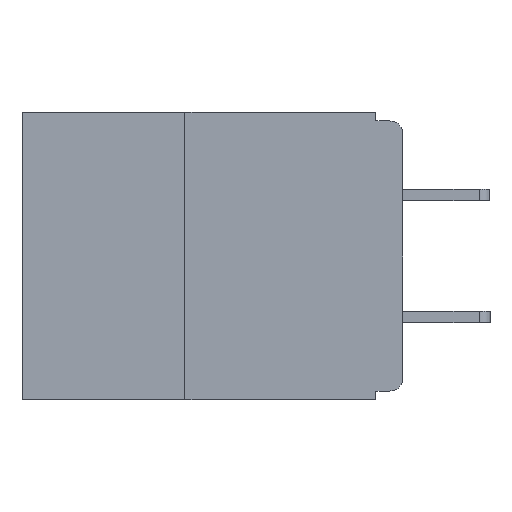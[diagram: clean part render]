
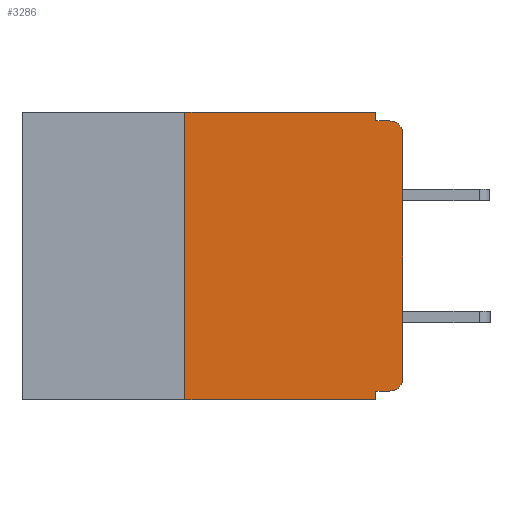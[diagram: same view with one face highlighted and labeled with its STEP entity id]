
A CAD part, left-side view. The second image highlights one B-rep face of the part: STEP entity #3286.
In plain terms, the highlighted planar face has unit normal (-1, 0, 0).
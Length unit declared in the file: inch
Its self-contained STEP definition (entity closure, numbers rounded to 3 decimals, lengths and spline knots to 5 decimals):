
#196 = CARTESIAN_POINT ( 'NONE',  ( 0., 0.031, 0. ) ) ;
#295 = EDGE_CURVE ( 'NONE', #16377, #27102, #6741, .T. ) ;
#444 = EDGE_CURVE ( 'NONE', #8592, #17327, #26393, .T. ) ;
#809 = DIRECTION ( 'NONE',  ( -1., 0., 0. ) ) ;
#1293 = VERTEX_POINT ( 'NONE', #15993 ) ;
#1761 = EDGE_CURVE ( 'NONE', #8592, #17050, #13873, .T. ) ;
#3118 = ORIENTED_EDGE ( 'NONE', *, *, #4079, .T. ) ;
#3286 = ADVANCED_FACE ( 'NONE', ( #9247 ), #17179, .F. ) ;
#4079 = EDGE_CURVE ( 'NONE', #17050, #16705, #19885, .T. ) ;
#4694 = ORIENTED_EDGE ( 'NONE', *, *, #1761, .T. ) ;
#5851 = CARTESIAN_POINT ( 'NONE',  ( 0., 0., 0. ) ) ;
#6332 = CARTESIAN_POINT ( 'NONE',  ( 0., 0., -0.025 ) ) ;
#6379 = CARTESIAN_POINT ( 'NONE',  ( 0., 0., -0.01 ) ) ;
#6396 = DIRECTION ( 'NONE',  ( 0., 0., -1. ) ) ;
#6573 = DIRECTION ( 'NONE',  ( 1., 0., 0. ) ) ;
#6720 = EDGE_LOOP ( 'NONE', ( #3118, #16031, #24712, #26273, #27797, #9269, #13804, #28202, #9662, #4694 ) ) ;
#6741 = LINE ( 'NONE', #27504, #24470 ) ;
#7081 = EDGE_CURVE ( 'NONE', #17327, #18658, #19704, .T. ) ;
#7130 = VERTEX_POINT ( 'NONE', #9991 ) ;
#7249 = VECTOR ( 'NONE', #15002, 39.37008 ) ;
#8592 = VERTEX_POINT ( 'NONE', #11400 ) ;
#9129 = CARTESIAN_POINT ( 'NONE',  ( 0., 0.031, -0.33 ) ) ;
#9247 = FACE_OUTER_BOUND ( 'NONE', #6720, .T. ) ;
#9269 = ORIENTED_EDGE ( 'NONE', *, *, #17254, .F. ) ;
#9607 = DIRECTION ( 'NONE',  ( 0., 0., -1. ) ) ;
#9662 = ORIENTED_EDGE ( 'NONE', *, *, #444, .F. ) ;
#9991 = CARTESIAN_POINT ( 'NONE',  ( 0., 0.015, -0.01 ) ) ;
#11129 = EDGE_CURVE ( 'NONE', #27102, #7130, #21011, .T. ) ;
#11400 = CARTESIAN_POINT ( 'NONE',  ( 0., 0.015, -0.32 ) ) ;
#11452 = VECTOR ( 'NONE', #14889, 39.37008 ) ;
#12587 = CARTESIAN_POINT ( 'NONE',  ( 0., 0.437, 0. ) ) ;
#13057 = CARTESIAN_POINT ( 'NONE',  ( 0., 0.437, 0. ) ) ;
#13178 = CARTESIAN_POINT ( 'NONE',  ( 0., 0.25, -0.33 ) ) ;
#13791 = VECTOR ( 'NONE', #26834, 39.37008 ) ;
#13804 = ORIENTED_EDGE ( 'NONE', *, *, #30881, .T. ) ;
#13873 = CIRCLE ( 'NONE', #25104, 0.015 ) ;
#13907 = EDGE_CURVE ( 'NONE', #1293, #16377, #20055, .T. ) ;
#14502 = AXIS2_PLACEMENT_3D ( 'NONE', #15390, #809, #17803 ) ;
#14889 = DIRECTION ( 'NONE',  ( 0., 0., 1. ) ) ;
#15002 = DIRECTION ( 'NONE',  ( 0., -1., 0. ) ) ;
#15288 = LINE ( 'NONE', #17187, #13791 ) ;
#15390 = CARTESIAN_POINT ( 'NONE',  ( 0., 0.015, -0.025 ) ) ;
#15820 = CARTESIAN_POINT ( 'NONE',  ( 0., 0., -0.32 ) ) ;
#15993 = CARTESIAN_POINT ( 'NONE',  ( 0., 0.25, 0. ) ) ;
#16031 = ORIENTED_EDGE ( 'NONE', *, *, #31030, .T. ) ;
#16377 = VERTEX_POINT ( 'NONE', #196 ) ;
#16412 = CIRCLE ( 'NONE', #14502, 0.015 ) ;
#16705 = VERTEX_POINT ( 'NONE', #6332 ) ;
#17050 = VERTEX_POINT ( 'NONE', #19587 ) ;
#17179 = PLANE ( 'NONE',  #22059 ) ;
#17187 = CARTESIAN_POINT ( 'NONE',  ( 0., 0.437, -0.33 ) ) ;
#17254 = EDGE_CURVE ( 'NONE', #20182, #1293, #30486, .T. ) ;
#17327 = VERTEX_POINT ( 'NONE', #23038 ) ;
#17803 = DIRECTION ( 'NONE',  ( 0., 0., -1. ) ) ;
#18658 = VERTEX_POINT ( 'NONE', #21382 ) ;
#18957 = VECTOR ( 'NONE', #9607, 39.37008 ) ;
#19587 = CARTESIAN_POINT ( 'NONE',  ( 0., 0., -0.305 ) ) ;
#19668 = DIRECTION ( 'NONE',  ( 0., 1., 0. ) ) ;
#19704 = LINE ( 'NONE', #9129, #18957 ) ;
#19885 = LINE ( 'NONE', #5851, #11452 ) ;
#19917 = VECTOR ( 'NONE', #19668, 39.37008 ) ;
#20055 = LINE ( 'NONE', #12587, #7249 ) ;
#20182 = VERTEX_POINT ( 'NONE', #20357 ) ;
#20357 = CARTESIAN_POINT ( 'NONE',  ( 0., 0.25, -0.33 ) ) ;
#21011 = LINE ( 'NONE', #6379, #26703 ) ;
#21261 = DIRECTION ( 'NONE',  ( -1., 0., 0. ) ) ;
#21382 = CARTESIAN_POINT ( 'NONE',  ( 0., 0.031, -0.33 ) ) ;
#22059 = AXIS2_PLACEMENT_3D ( 'NONE', #13057, #6573, #6396 ) ;
#23038 = CARTESIAN_POINT ( 'NONE',  ( 0., 0.031, -0.32 ) ) ;
#24038 = VECTOR ( 'NONE', #30045, 39.37008 ) ;
#24470 = VECTOR ( 'NONE', #29780, 39.37008 ) ;
#24712 = ORIENTED_EDGE ( 'NONE', *, *, #11129, .F. ) ;
#25104 = AXIS2_PLACEMENT_3D ( 'NONE', #25487, #21261, #25636 ) ;
#25487 = CARTESIAN_POINT ( 'NONE',  ( 0., 0.015, -0.305 ) ) ;
#25636 = DIRECTION ( 'NONE',  ( 0., 0., -1. ) ) ;
#25730 = DIRECTION ( 'NONE',  ( 0., -1., 0. ) ) ;
#26273 = ORIENTED_EDGE ( 'NONE', *, *, #295, .F. ) ;
#26393 = LINE ( 'NONE', #15820, #19917 ) ;
#26703 = VECTOR ( 'NONE', #25730, 39.37008 ) ;
#26834 = DIRECTION ( 'NONE',  ( 0., -1., 0. ) ) ;
#27102 = VERTEX_POINT ( 'NONE', #29825 ) ;
#27504 = CARTESIAN_POINT ( 'NONE',  ( 0., 0.031, 0. ) ) ;
#27797 = ORIENTED_EDGE ( 'NONE', *, *, #13907, .F. ) ;
#28202 = ORIENTED_EDGE ( 'NONE', *, *, #7081, .F. ) ;
#29780 = DIRECTION ( 'NONE',  ( 0., 0., -1. ) ) ;
#29825 = CARTESIAN_POINT ( 'NONE',  ( 0., 0.031, -0.01 ) ) ;
#30045 = DIRECTION ( 'NONE',  ( 0., 0., 1. ) ) ;
#30486 = LINE ( 'NONE', #13178, #24038 ) ;
#30881 = EDGE_CURVE ( 'NONE', #20182, #18658, #15288, .T. ) ;
#31030 = EDGE_CURVE ( 'NONE', #16705, #7130, #16412, .T. ) ;
